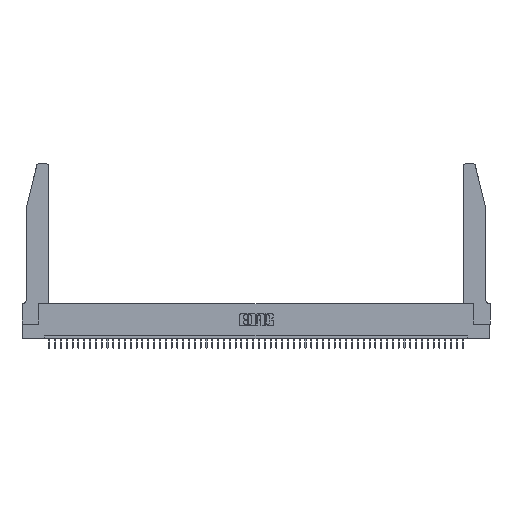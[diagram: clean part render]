
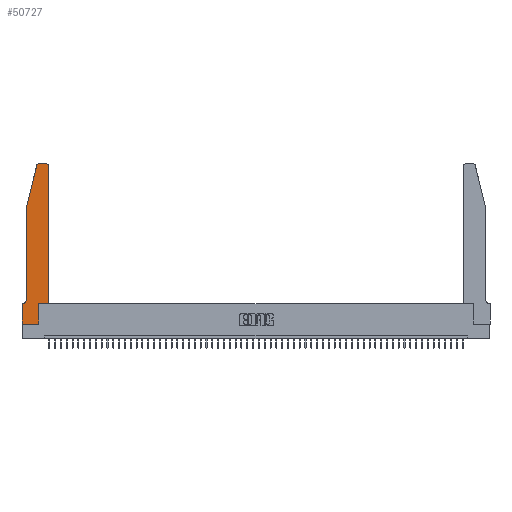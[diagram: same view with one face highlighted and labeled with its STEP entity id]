
A CAD part, top view. The second image highlights one B-rep face of the part: STEP entity #50727.
In plain terms, the highlighted planar face has unit normal (0, 0, 1).
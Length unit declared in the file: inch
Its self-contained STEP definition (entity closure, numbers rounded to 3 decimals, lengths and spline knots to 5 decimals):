
#468 = VECTOR ( 'NONE', #9441, 39.37008 ) ;
#926 = CARTESIAN_POINT ( 'NONE',  ( 0.0755, 2., 0.37 ) ) ;
#1424 = CARTESIAN_POINT ( 'NONE',  ( 0.0755, 2., 0.37 ) ) ;
#2459 = ORIENTED_EDGE ( 'NONE', *, *, #5178, .T. ) ;
#2703 = CARTESIAN_POINT ( 'NONE',  ( 0., 0., 0.37 ) ) ;
#2970 = ORIENTED_EDGE ( 'NONE', *, *, #43704, .T. ) ;
#3759 = AXIS2_PLACEMENT_3D ( 'NONE', #12918, #51099, #4355 ) ;
#4355 = DIRECTION ( 'NONE',  ( 1., 0., 0. ) ) ;
#5178 = EDGE_CURVE ( 'NONE', #28848, #54549, #51046, .T. ) ;
#5298 = FACE_OUTER_BOUND ( 'NONE', #53076, .T. ) ;
#6427 = EDGE_CURVE ( 'NONE', #51624, #39415, #13291, .T. ) ;
#6511 = EDGE_CURVE ( 'NONE', #54549, #33726, #40473, .T. ) ;
#8102 = CARTESIAN_POINT ( 'NONE',  ( 0.4505, 2.72, 0.37 ) ) ;
#9005 = DIRECTION ( 'NONE',  ( -1., 0., 0. ) ) ;
#9441 = DIRECTION ( 'NONE',  ( 0., -1., 0. ) ) ;
#11644 = DIRECTION ( 'NONE',  ( 0., 0., 1. ) ) ;
#11656 = VECTOR ( 'NONE', #35204, 39.37008 ) ;
#11683 = EDGE_CURVE ( 'NONE', #12032, #51624, #26613, .T. ) ;
#12032 = VERTEX_POINT ( 'NONE', #19168 ) ;
#12298 = LINE ( 'NONE', #27380, #32771 ) ;
#12563 = PLANE ( 'NONE',  #3759 ) ;
#12643 = VECTOR ( 'NONE', #15868, 39.37008 ) ;
#12918 = CARTESIAN_POINT ( 'NONE',  ( 0., 0.35, 0.37 ) ) ;
#13291 = CIRCLE ( 'NONE', #25555, 0.03 ) ;
#14014 = ORIENTED_EDGE ( 'NONE', *, *, #6427, .T. ) ;
#14594 = ORIENTED_EDGE ( 'NONE', *, *, #29759, .T. ) ;
#14772 = CARTESIAN_POINT ( 'NONE',  ( 0.284, 2.72, 0.37 ) ) ;
#14973 = DIRECTION ( 'NONE',  ( 0., 1., 0. ) ) ;
#14980 = EDGE_CURVE ( 'NONE', #35237, #28848, #15860, .T. ) ;
#15860 = LINE ( 'NONE', #1424, #468 ) ;
#15868 = DIRECTION ( 'NONE',  ( -1., 0., 0. ) ) ;
#15927 = CARTESIAN_POINT ( 'NONE',  ( 0.4205, 2.72, 0.37 ) ) ;
#15962 = VECTOR ( 'NONE', #9005, 39.37008 ) ;
#16121 = ORIENTED_EDGE ( 'NONE', *, *, #11683, .T. ) ;
#16502 = EDGE_CURVE ( 'NONE', #21409, #17608, #44111, .T. ) ;
#16700 = CARTESIAN_POINT ( 'NONE',  ( 0.0055, 0.42, 0.37 ) ) ;
#16880 = VERTEX_POINT ( 'NONE', #41530 ) ;
#17608 = VERTEX_POINT ( 'NONE', #38670 ) ;
#17660 = CARTESIAN_POINT ( 'NONE',  ( 0.0055, 0.35, 0.37 ) ) ;
#18998 = ORIENTED_EDGE ( 'NONE', *, *, #33788, .T. ) ;
#19168 = CARTESIAN_POINT ( 'NONE',  ( 0.4505, 0.35, 0.37 ) ) ;
#19185 = AXIS2_PLACEMENT_3D ( 'NONE', #14772, #44477, #53012 ) ;
#20628 = CARTESIAN_POINT ( 'NONE',  ( 0., 0., 0.37 ) ) ;
#21409 = VERTEX_POINT ( 'NONE', #20628 ) ;
#22224 = ORIENTED_EDGE ( 'NONE', *, *, #22937, .T. ) ;
#22886 = LINE ( 'NONE', #26188, #11656 ) ;
#22937 = EDGE_CURVE ( 'NONE', #33726, #21409, #22980, .T. ) ;
#22980 = LINE ( 'NONE', #52985, #32931 ) ;
#24630 = DIRECTION ( 'NONE',  ( 1., 0., 0. ) ) ;
#25555 = AXIS2_PLACEMENT_3D ( 'NONE', #15927, #11644, #24630 ) ;
#25976 = VECTOR ( 'NONE', #31935, 39.37008 ) ;
#26177 = CARTESIAN_POINT ( 'NONE',  ( 0.2865, 0.35, 0.37 ) ) ;
#26188 = CARTESIAN_POINT ( 'NONE',  ( 0.0755, 2., 0.37 ) ) ;
#26613 = LINE ( 'NONE', #44427, #25976 ) ;
#27380 = CARTESIAN_POINT ( 'NONE',  ( 0.4505, 0.35, 0.37 ) ) ;
#28093 = DIRECTION ( 'NONE',  ( 1., 0., 0. ) ) ;
#28848 = VERTEX_POINT ( 'NONE', #42077 ) ;
#28885 = VECTOR ( 'NONE', #14973, 39.37008 ) ;
#29759 = EDGE_CURVE ( 'NONE', #39415, #41147, #38418, .T. ) ;
#30576 = VERTEX_POINT ( 'NONE', #26177 ) ;
#30747 = CARTESIAN_POINT ( 'NONE',  ( 0., 0.35, 0.37 ) ) ;
#31836 = CARTESIAN_POINT ( 'NONE',  ( 0.4205, 2.75, 0.37 ) ) ;
#31935 = DIRECTION ( 'NONE',  ( 0., 1., 0. ) ) ;
#32771 = VECTOR ( 'NONE', #52653, 39.37008 ) ;
#32931 = VECTOR ( 'NONE', #40317, 39.37008 ) ;
#33726 = VERTEX_POINT ( 'NONE', #30747 ) ;
#33788 = EDGE_CURVE ( 'NONE', #30576, #12032, #12298, .T. ) ;
#34592 = CARTESIAN_POINT ( 'NONE',  ( 0.284, 2.75, 0.37 ) ) ;
#35204 = DIRECTION ( 'NONE',  ( -0.239, -0.971, 0. ) ) ;
#35237 = VERTEX_POINT ( 'NONE', #926 ) ;
#37263 = AXIS2_PLACEMENT_3D ( 'NONE', #16700, #37329, #47637 ) ;
#37329 = DIRECTION ( 'NONE',  ( 0., 0., -1. ) ) ;
#37869 = ORIENTED_EDGE ( 'NONE', *, *, #16502, .T. ) ;
#38418 = LINE ( 'NONE', #39156, #15962 ) ;
#38670 = CARTESIAN_POINT ( 'NONE',  ( 0.2865, 0., 0.37 ) ) ;
#39156 = CARTESIAN_POINT ( 'NONE',  ( 0.2605, 2.75, 0.37 ) ) ;
#39415 = VERTEX_POINT ( 'NONE', #31836 ) ;
#39944 = CARTESIAN_POINT ( 'NONE',  ( 0.2865, 0.35, 0.37 ) ) ;
#40317 = DIRECTION ( 'NONE',  ( 0., -1., 0. ) ) ;
#40473 = LINE ( 'NONE', #53700, #12643 ) ;
#40817 = VECTOR ( 'NONE', #28093, 39.37008 ) ;
#41147 = VERTEX_POINT ( 'NONE', #34592 ) ;
#41530 = CARTESIAN_POINT ( 'NONE',  ( 0.25487, 2.72718, 0.37 ) ) ;
#42077 = CARTESIAN_POINT ( 'NONE',  ( 0.0755, 0.42, 0.37 ) ) ;
#42111 = ORIENTED_EDGE ( 'NONE', *, *, #53447, .T. ) ;
#43704 = EDGE_CURVE ( 'NONE', #41147, #16880, #49623, .T. ) ;
#44111 = LINE ( 'NONE', #2703, #40817 ) ;
#44427 = CARTESIAN_POINT ( 'NONE',  ( 0.4505, 0.35, 0.37 ) ) ;
#44477 = DIRECTION ( 'NONE',  ( 0., 0., 1. ) ) ;
#46269 = ORIENTED_EDGE ( 'NONE', *, *, #14980, .T. ) ;
#47637 = DIRECTION ( 'NONE',  ( -1., 0., 0. ) ) ;
#49535 = LINE ( 'NONE', #39944, #28885 ) ;
#49623 = CIRCLE ( 'NONE', #19185, 0.03 ) ;
#50727 = ADVANCED_FACE ( 'NONE', ( #5298 ), #12563, .T. ) ;
#51046 = CIRCLE ( 'NONE', #37263, 0.07 ) ;
#51099 = DIRECTION ( 'NONE',  ( 0., 0., 1. ) ) ;
#51624 = VERTEX_POINT ( 'NONE', #8102 ) ;
#51705 = ORIENTED_EDGE ( 'NONE', *, *, #6511, .T. ) ;
#52653 = DIRECTION ( 'NONE',  ( 1., 0., 0. ) ) ;
#52985 = CARTESIAN_POINT ( 'NONE',  ( 0., 0., 0.37 ) ) ;
#53012 = DIRECTION ( 'NONE',  ( 1., 0., 0. ) ) ;
#53076 = EDGE_LOOP ( 'NONE', ( #14594, #2970, #54974, #46269, #2459, #51705, #22224, #37869, #42111, #18998, #16121, #14014 ) ) ;
#53447 = EDGE_CURVE ( 'NONE', #17608, #30576, #49535, .T. ) ;
#53700 = CARTESIAN_POINT ( 'NONE',  ( 0.0755, 0.35, 0.37 ) ) ;
#54026 = EDGE_CURVE ( 'NONE', #16880, #35237, #22886, .T. ) ;
#54549 = VERTEX_POINT ( 'NONE', #17660 ) ;
#54974 = ORIENTED_EDGE ( 'NONE', *, *, #54026, .T. ) ;
